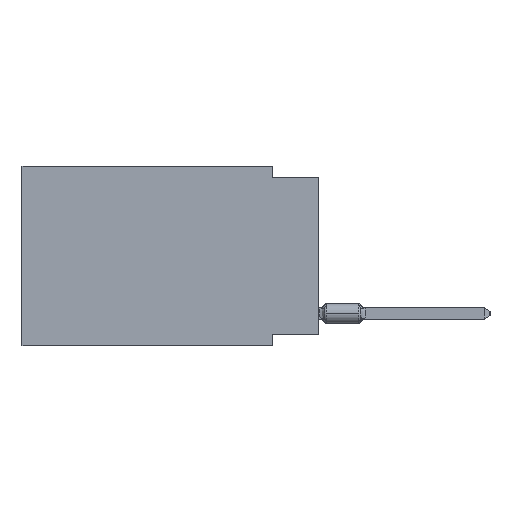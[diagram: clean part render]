
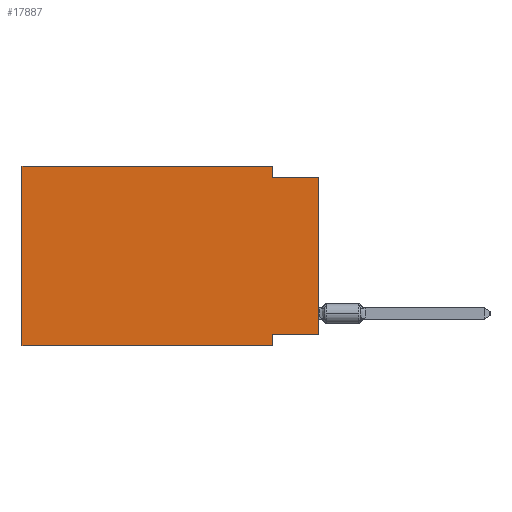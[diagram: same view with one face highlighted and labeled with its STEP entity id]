
A CAD part, left-side view. The second image highlights one B-rep face of the part: STEP entity #17887.
In plain terms, the highlighted planar face has unit normal (-1, 0, 0).
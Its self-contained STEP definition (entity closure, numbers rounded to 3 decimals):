
#1020 = VECTOR ( 'NONE', #31233, 1000. ) ;
#1031 = VERTEX_POINT ( 'NONE', #22478 ) ;
#1277 = CARTESIAN_POINT ( 'NONE',  ( 0., 0., -9.271 ) ) ;
#1709 = CARTESIAN_POINT ( 'NONE',  ( 0., 0., -0.635 ) ) ;
#2199 = DIRECTION ( 'NONE',  ( 0., 0., -1. ) ) ;
#2715 = EDGE_CURVE ( 'NONE', #26819, #26910, #15739, .T. ) ;
#2804 = LINE ( 'NONE', #8131, #7031 ) ;
#2886 = VECTOR ( 'NONE', #2199, 1000. ) ;
#3703 = ORIENTED_EDGE ( 'NONE', *, *, #3726, .F. ) ;
#3726 = EDGE_CURVE ( 'NONE', #7081, #4893, #17547, .T. ) ;
#3915 = CARTESIAN_POINT ( 'NONE',  ( 0., 0., 0. ) ) ;
#4893 = VERTEX_POINT ( 'NONE', #10270 ) ;
#5340 = VECTOR ( 'NONE', #6492, 1000. ) ;
#5357 = LINE ( 'NONE', #29785, #11848 ) ;
#5863 = ORIENTED_EDGE ( 'NONE', *, *, #2715, .F. ) ;
#6121 = ORIENTED_EDGE ( 'NONE', *, *, #9247, .F. ) ;
#6380 = ORIENTED_EDGE ( 'NONE', *, *, #11399, .F. ) ;
#6492 = DIRECTION ( 'NONE',  ( 0., 0., 1. ) ) ;
#7031 = VECTOR ( 'NONE', #17997, 1000. ) ;
#7081 = VERTEX_POINT ( 'NONE', #23773 ) ;
#7365 = LINE ( 'NONE', #11745, #2886 ) ;
#8131 = CARTESIAN_POINT ( 'NONE',  ( 0., 16.383, -9.906 ) ) ;
#8696 = PLANE ( 'NONE',  #9052 ) ;
#9052 = AXIS2_PLACEMENT_3D ( 'NONE', #26467, #23568, #21627 ) ;
#9134 = VECTOR ( 'NONE', #29844, 1000. ) ;
#9247 = EDGE_CURVE ( 'NONE', #1031, #20264, #7365, .T. ) ;
#9901 = ORIENTED_EDGE ( 'NONE', *, *, #18651, .T. ) ;
#10270 = CARTESIAN_POINT ( 'NONE',  ( 0., 2.54, -0.635 ) ) ;
#10887 = CARTESIAN_POINT ( 'NONE',  ( 0., 16.383, 0. ) ) ;
#11399 = EDGE_CURVE ( 'NONE', #28370, #1031, #18103, .T. ) ;
#11745 = CARTESIAN_POINT ( 'NONE',  ( 0., 2.54, -9.906 ) ) ;
#11848 = VECTOR ( 'NONE', #27025, 1000. ) ;
#12182 = EDGE_CURVE ( 'NONE', #28370, #29822, #31222, .T. ) ;
#15739 = LINE ( 'NONE', #10887, #24636 ) ;
#16490 = CARTESIAN_POINT ( 'NONE',  ( 0., 2.54, -9.906 ) ) ;
#17547 = LINE ( 'NONE', #22561, #9134 ) ;
#17887 = ADVANCED_FACE ( 'NONE', ( #19041 ), #8696, .F. ) ;
#17997 = DIRECTION ( 'NONE',  ( 0., -1., 0. ) ) ;
#18103 = LINE ( 'NONE', #1277, #19234 ) ;
#18651 = EDGE_CURVE ( 'NONE', #26819, #20264, #2804, .T. ) ;
#19041 = FACE_OUTER_BOUND ( 'NONE', #23942, .T. ) ;
#19234 = VECTOR ( 'NONE', #25861, 1000. ) ;
#20264 = VERTEX_POINT ( 'NONE', #16490 ) ;
#20393 = ORIENTED_EDGE ( 'NONE', *, *, #12182, .T. ) ;
#20924 = CARTESIAN_POINT ( 'NONE',  ( 0., 0., -9.271 ) ) ;
#21367 = CARTESIAN_POINT ( 'NONE',  ( 0., 0., -0.635 ) ) ;
#21627 = DIRECTION ( 'NONE',  ( 0., 0., -1. ) ) ;
#21704 = LINE ( 'NONE', #21367, #1020 ) ;
#22319 = ORIENTED_EDGE ( 'NONE', *, *, #22532, .F. ) ;
#22478 = CARTESIAN_POINT ( 'NONE',  ( 0., 2.54, -9.271 ) ) ;
#22532 = EDGE_CURVE ( 'NONE', #4893, #29822, #21704, .T. ) ;
#22561 = CARTESIAN_POINT ( 'NONE',  ( 0., 2.54, 0. ) ) ;
#22705 = DIRECTION ( 'NONE',  ( 0., 0., 1. ) ) ;
#22879 = CARTESIAN_POINT ( 'NONE',  ( 0., 16.383, 0. ) ) ;
#23568 = DIRECTION ( 'NONE',  ( 1., 0., 0. ) ) ;
#23773 = CARTESIAN_POINT ( 'NONE',  ( 0., 2.54, 0. ) ) ;
#23837 = EDGE_CURVE ( 'NONE', #26910, #7081, #5357, .T. ) ;
#23942 = EDGE_LOOP ( 'NONE', ( #20393, #22319, #3703, #24615, #5863, #9901, #6121, #6380 ) ) ;
#24615 = ORIENTED_EDGE ( 'NONE', *, *, #23837, .F. ) ;
#24636 = VECTOR ( 'NONE', #22705, 1000. ) ;
#25861 = DIRECTION ( 'NONE',  ( 0., 1., 0. ) ) ;
#26467 = CARTESIAN_POINT ( 'NONE',  ( 0., 16.383, 0. ) ) ;
#26819 = VERTEX_POINT ( 'NONE', #31630 ) ;
#26910 = VERTEX_POINT ( 'NONE', #22879 ) ;
#27025 = DIRECTION ( 'NONE',  ( 0., -1., 0. ) ) ;
#28370 = VERTEX_POINT ( 'NONE', #20924 ) ;
#29785 = CARTESIAN_POINT ( 'NONE',  ( 0., 16.383, 0. ) ) ;
#29822 = VERTEX_POINT ( 'NONE', #1709 ) ;
#29844 = DIRECTION ( 'NONE',  ( 0., 0., -1. ) ) ;
#31222 = LINE ( 'NONE', #3915, #5340 ) ;
#31233 = DIRECTION ( 'NONE',  ( 0., -1., 0. ) ) ;
#31630 = CARTESIAN_POINT ( 'NONE',  ( 0., 16.383, -9.906 ) ) ;
